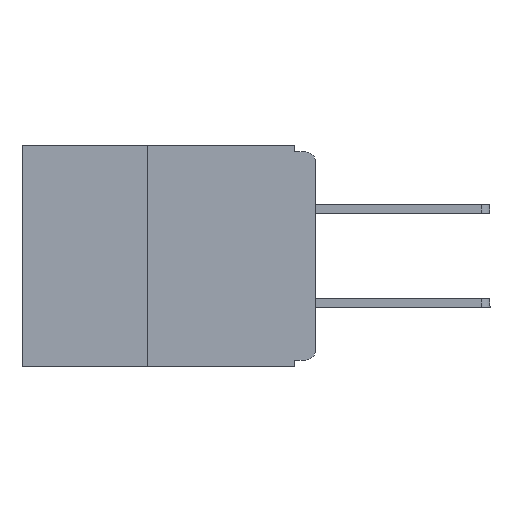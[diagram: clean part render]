
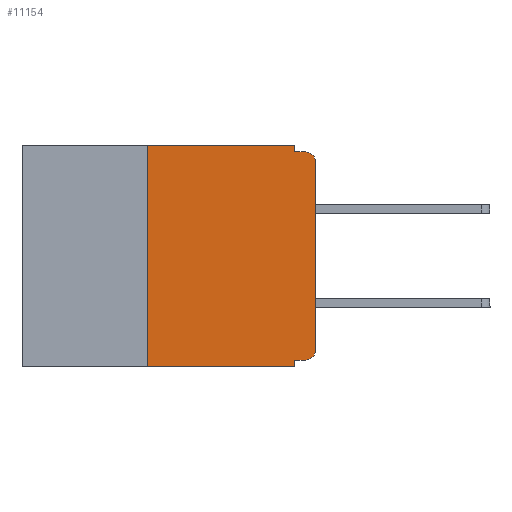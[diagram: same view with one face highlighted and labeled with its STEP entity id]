
A CAD part, left-side view. The second image highlights one B-rep face of the part: STEP entity #11154.
In plain terms, the highlighted planar face has unit normal (-1, 0, 0).
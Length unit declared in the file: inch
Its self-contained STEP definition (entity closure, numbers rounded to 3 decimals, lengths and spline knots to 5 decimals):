
#106 = VECTOR ( 'NONE', #18313, 39.37008 ) ;
#298 = CARTESIAN_POINT ( 'NONE',  ( 0., 0., 0. ) ) ;
#393 = VECTOR ( 'NONE', #16185, 39.37008 ) ;
#889 = CIRCLE ( 'NONE', #24060, 0.015 ) ;
#1338 = VERTEX_POINT ( 'NONE', #16471 ) ;
#1805 = FACE_OUTER_BOUND ( 'NONE', #13452, .T. ) ;
#1859 = CARTESIAN_POINT ( 'NONE',  ( 0., 0.437, 0. ) ) ;
#1866 = EDGE_CURVE ( 'NONE', #14252, #19664, #1952, .T. ) ;
#1952 = LINE ( 'NONE', #19830, #12320 ) ;
#2143 = CARTESIAN_POINT ( 'NONE',  ( 0., 0.015, -0.32 ) ) ;
#2259 = VERTEX_POINT ( 'NONE', #21379 ) ;
#2313 = ORIENTED_EDGE ( 'NONE', *, *, #1866, .F. ) ;
#2851 = VERTEX_POINT ( 'NONE', #22315 ) ;
#3062 = VECTOR ( 'NONE', #8171, 39.37008 ) ;
#3813 = AXIS2_PLACEMENT_3D ( 'NONE', #1859, #20359, #8164 ) ;
#4166 = CARTESIAN_POINT ( 'NONE',  ( 0., 0.031, -0.32 ) ) ;
#4614 = EDGE_CURVE ( 'NONE', #13526, #2851, #24519, .T. ) ;
#5293 = ORIENTED_EDGE ( 'NONE', *, *, #17705, .F. ) ;
#6209 = CARTESIAN_POINT ( 'NONE',  ( 0., 0.031, 0. ) ) ;
#6219 = CIRCLE ( 'NONE', #17537, 0.015 ) ;
#6436 = CARTESIAN_POINT ( 'NONE',  ( 0., 0.015, -0.025 ) ) ;
#6597 = ORIENTED_EDGE ( 'NONE', *, *, #13639, .T. ) ;
#6617 = LINE ( 'NONE', #8121, #393 ) ;
#7722 = VERTEX_POINT ( 'NONE', #11157 ) ;
#7867 = DIRECTION ( 'NONE',  ( -1., 0., 0. ) ) ;
#8121 = CARTESIAN_POINT ( 'NONE',  ( 0., 0.437, -0.33 ) ) ;
#8131 = LINE ( 'NONE', #6209, #12922 ) ;
#8164 = DIRECTION ( 'NONE',  ( 0., 0., -1. ) ) ;
#8171 = DIRECTION ( 'NONE',  ( 0., -1., 0. ) ) ;
#8284 = DIRECTION ( 'NONE',  ( 0., 0., -1. ) ) ;
#8503 = DIRECTION ( 'NONE',  ( 0., 0., -1. ) ) ;
#8564 = ORIENTED_EDGE ( 'NONE', *, *, #19771, .T. ) ;
#8760 = CARTESIAN_POINT ( 'NONE',  ( 0., 0.437, 0. ) ) ;
#9657 = CARTESIAN_POINT ( 'NONE',  ( 0., 0.031, -0.33 ) ) ;
#9668 = CARTESIAN_POINT ( 'NONE',  ( 0., 0.031, -0.33 ) ) ;
#10163 = PLANE ( 'NONE',  #3813 ) ;
#11154 = ADVANCED_FACE ( 'NONE', ( #1805 ), #10163, .F. ) ;
#11157 = CARTESIAN_POINT ( 'NONE',  ( 0., 0.015, -0.01 ) ) ;
#11525 = LINE ( 'NONE', #9657, #16236 ) ;
#12263 = EDGE_CURVE ( 'NONE', #19664, #26022, #11525, .T. ) ;
#12320 = VECTOR ( 'NONE', #26172, 39.37008 ) ;
#12922 = VECTOR ( 'NONE', #8284, 39.37008 ) ;
#12954 = EDGE_CURVE ( 'NONE', #15048, #7722, #16530, .T. ) ;
#13452 = EDGE_LOOP ( 'NONE', ( #8564, #19400, #25108, #5293, #16144, #21497, #6597, #23278, #2313, #23872 ) ) ;
#13526 = VERTEX_POINT ( 'NONE', #15934 ) ;
#13639 = EDGE_CURVE ( 'NONE', #19714, #26022, #6617, .T. ) ;
#14252 = VERTEX_POINT ( 'NONE', #2143 ) ;
#14254 = CARTESIAN_POINT ( 'NONE',  ( 0., 0., -0.01 ) ) ;
#15048 = VERTEX_POINT ( 'NONE', #24816 ) ;
#15392 = VECTOR ( 'NONE', #23090, 39.37008 ) ;
#15728 = DIRECTION ( 'NONE',  ( 0., 0., -1. ) ) ;
#15934 = CARTESIAN_POINT ( 'NONE',  ( 0., 0.25, 0. ) ) ;
#16144 = ORIENTED_EDGE ( 'NONE', *, *, #4614, .F. ) ;
#16185 = DIRECTION ( 'NONE',  ( 0., -1., 0. ) ) ;
#16236 = VECTOR ( 'NONE', #15728, 39.37008 ) ;
#16308 = EDGE_CURVE ( 'NONE', #19714, #13526, #25846, .T. ) ;
#16471 = CARTESIAN_POINT ( 'NONE',  ( 0., 0., -0.025 ) ) ;
#16530 = LINE ( 'NONE', #14254, #106 ) ;
#17249 = LINE ( 'NONE', #298, #22485 ) ;
#17537 = AXIS2_PLACEMENT_3D ( 'NONE', #6436, #20678, #8503 ) ;
#17705 = EDGE_CURVE ( 'NONE', #2851, #15048, #8131, .T. ) ;
#18313 = DIRECTION ( 'NONE',  ( 0., -1., 0. ) ) ;
#18893 = EDGE_CURVE ( 'NONE', #14252, #2259, #889, .T. ) ;
#19400 = ORIENTED_EDGE ( 'NONE', *, *, #22801, .T. ) ;
#19664 = VERTEX_POINT ( 'NONE', #4166 ) ;
#19714 = VERTEX_POINT ( 'NONE', #20669 ) ;
#19771 = EDGE_CURVE ( 'NONE', #2259, #1338, #17249, .T. ) ;
#19830 = CARTESIAN_POINT ( 'NONE',  ( 0., 0., -0.32 ) ) ;
#20072 = CARTESIAN_POINT ( 'NONE',  ( 0., 0.015, -0.305 ) ) ;
#20359 = DIRECTION ( 'NONE',  ( 1., 0., 0. ) ) ;
#20669 = CARTESIAN_POINT ( 'NONE',  ( 0., 0.25, -0.33 ) ) ;
#20678 = DIRECTION ( 'NONE',  ( -1., 0., 0. ) ) ;
#21195 = CARTESIAN_POINT ( 'NONE',  ( 0., 0.25, -0.33 ) ) ;
#21379 = CARTESIAN_POINT ( 'NONE',  ( 0., 0., -0.305 ) ) ;
#21497 = ORIENTED_EDGE ( 'NONE', *, *, #16308, .F. ) ;
#21977 = DIRECTION ( 'NONE',  ( 0., 0., -1. ) ) ;
#22315 = CARTESIAN_POINT ( 'NONE',  ( 0., 0.031, 0. ) ) ;
#22485 = VECTOR ( 'NONE', #22642, 39.37008 ) ;
#22642 = DIRECTION ( 'NONE',  ( 0., 0., 1. ) ) ;
#22801 = EDGE_CURVE ( 'NONE', #1338, #7722, #6219, .T. ) ;
#23090 = DIRECTION ( 'NONE',  ( 0., 0., 1. ) ) ;
#23278 = ORIENTED_EDGE ( 'NONE', *, *, #12263, .F. ) ;
#23872 = ORIENTED_EDGE ( 'NONE', *, *, #18893, .T. ) ;
#24060 = AXIS2_PLACEMENT_3D ( 'NONE', #20072, #7867, #21977 ) ;
#24519 = LINE ( 'NONE', #8760, #3062 ) ;
#24816 = CARTESIAN_POINT ( 'NONE',  ( 0., 0.031, -0.01 ) ) ;
#25108 = ORIENTED_EDGE ( 'NONE', *, *, #12954, .F. ) ;
#25846 = LINE ( 'NONE', #21195, #15392 ) ;
#26022 = VERTEX_POINT ( 'NONE', #9668 ) ;
#26172 = DIRECTION ( 'NONE',  ( 0., 1., 0. ) ) ;
